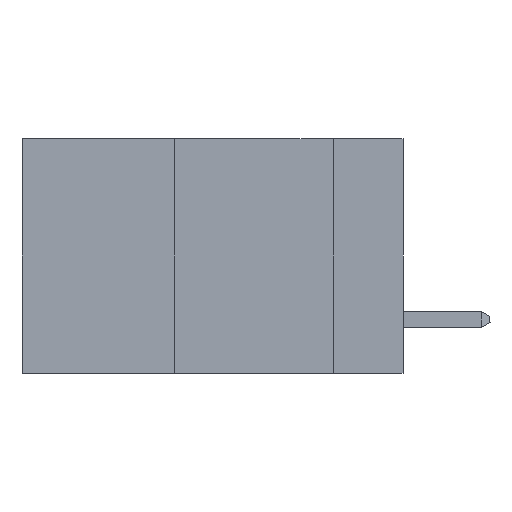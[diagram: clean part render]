
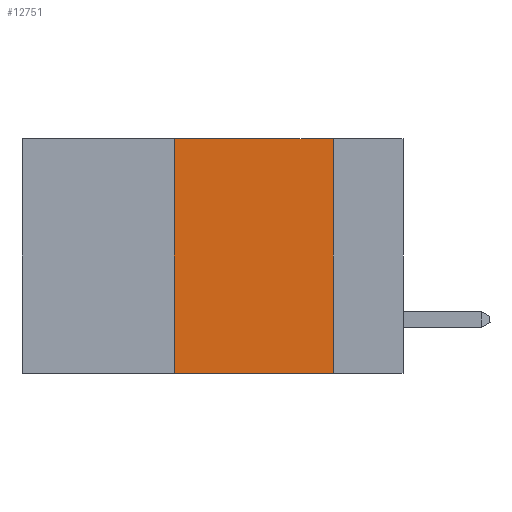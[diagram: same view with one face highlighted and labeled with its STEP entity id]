
A CAD part, left-side view. The second image highlights one B-rep face of the part: STEP entity #12751.
In plain terms, the highlighted planar face has unit normal (-1, 0, 0).
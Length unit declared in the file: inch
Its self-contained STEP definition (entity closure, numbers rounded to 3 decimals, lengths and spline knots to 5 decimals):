
#768 = CARTESIAN_POINT ( 'NONE',  ( 0., 0.6, 0. ) ) ;
#822 = ORIENTED_EDGE ( 'NONE', *, *, #4117, .F. ) ;
#1665 = CARTESIAN_POINT ( 'NONE',  ( 0., 0.6, -0.37 ) ) ;
#2827 = CARTESIAN_POINT ( 'NONE',  ( 0., 0.11, 0. ) ) ;
#3365 = LINE ( 'NONE', #6425, #13135 ) ;
#3544 = DIRECTION ( 'NONE',  ( 0., 0., -1. ) ) ;
#3588 = EDGE_CURVE ( 'NONE', #16042, #13748, #13188, .T. ) ;
#3721 = AXIS2_PLACEMENT_3D ( 'NONE', #768, #12490, #3544 ) ;
#4117 = EDGE_CURVE ( 'NONE', #14989, #13748, #6024, .T. ) ;
#4357 = CARTESIAN_POINT ( 'NONE',  ( 0., 0.36, -0.37 ) ) ;
#4400 = VECTOR ( 'NONE', #6203, 39.37008 ) ;
#4547 = EDGE_LOOP ( 'NONE', ( #822, #14971, #11109, #13956 ) ) ;
#4893 = EDGE_CURVE ( 'NONE', #6533, #14989, #3365, .T. ) ;
#4999 = LINE ( 'NONE', #5796, #5401 ) ;
#5363 = EDGE_CURVE ( 'NONE', #16042, #6533, #4999, .T. ) ;
#5401 = VECTOR ( 'NONE', #5740, 39.37008 ) ;
#5740 = DIRECTION ( 'NONE',  ( 0., 0., 1. ) ) ;
#5796 = CARTESIAN_POINT ( 'NONE',  ( 0., 0.36, 0. ) ) ;
#6024 = LINE ( 'NONE', #7689, #4400 ) ;
#6203 = DIRECTION ( 'NONE',  ( 0., 0., -1. ) ) ;
#6425 = CARTESIAN_POINT ( 'NONE',  ( 0., 0.6, 0. ) ) ;
#6533 = VERTEX_POINT ( 'NONE', #10227 ) ;
#6868 = VECTOR ( 'NONE', #11911, 39.37008 ) ;
#7689 = CARTESIAN_POINT ( 'NONE',  ( 0., 0.11, 0. ) ) ;
#7849 = DIRECTION ( 'NONE',  ( 0., -1., 0. ) ) ;
#10227 = CARTESIAN_POINT ( 'NONE',  ( 0., 0.36, 0. ) ) ;
#11109 = ORIENTED_EDGE ( 'NONE', *, *, #5363, .F. ) ;
#11911 = DIRECTION ( 'NONE',  ( 0., -1., 0. ) ) ;
#12199 = CARTESIAN_POINT ( 'NONE',  ( 0., 0.11, -0.37 ) ) ;
#12490 = DIRECTION ( 'NONE',  ( 1., 0., 0. ) ) ;
#12751 = ADVANCED_FACE ( 'NONE', ( #15791 ), #15242, .F. ) ;
#13135 = VECTOR ( 'NONE', #7849, 39.37008 ) ;
#13188 = LINE ( 'NONE', #1665, #6868 ) ;
#13748 = VERTEX_POINT ( 'NONE', #12199 ) ;
#13956 = ORIENTED_EDGE ( 'NONE', *, *, #3588, .T. ) ;
#14971 = ORIENTED_EDGE ( 'NONE', *, *, #4893, .F. ) ;
#14989 = VERTEX_POINT ( 'NONE', #2827 ) ;
#15242 = PLANE ( 'NONE',  #3721 ) ;
#15791 = FACE_OUTER_BOUND ( 'NONE', #4547, .T. ) ;
#16042 = VERTEX_POINT ( 'NONE', #4357 ) ;
